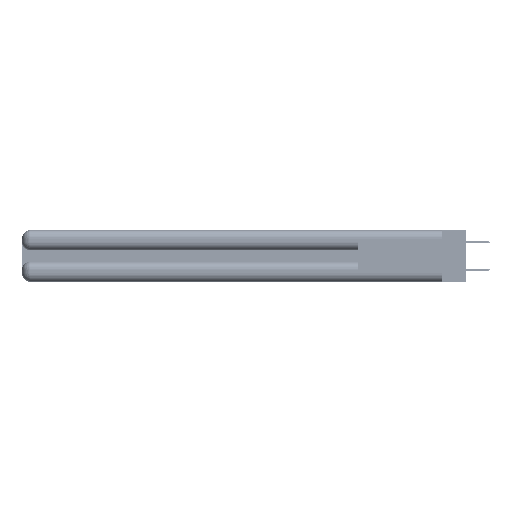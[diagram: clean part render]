
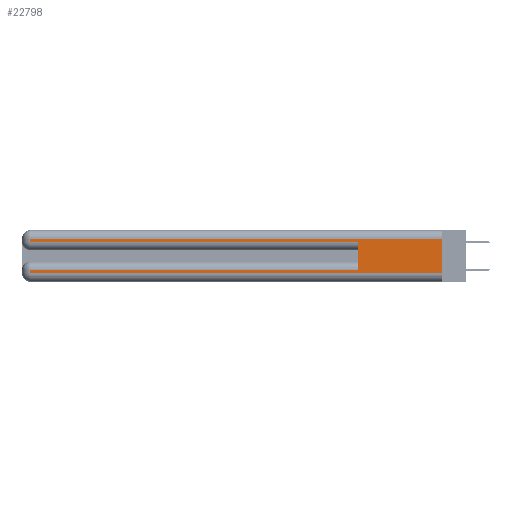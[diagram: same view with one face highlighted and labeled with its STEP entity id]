
A CAD part, left-side view. The second image highlights one B-rep face of the part: STEP entity #22798.
In plain terms, the highlighted planar face has unit normal (-1, 0, 0).
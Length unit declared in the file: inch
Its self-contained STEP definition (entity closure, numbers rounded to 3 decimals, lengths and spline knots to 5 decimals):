
#165 = CARTESIAN_POINT ( 'NONE',  ( 0., 2.94, 0.285 ) ) ;
#1578 = ORIENTED_EDGE ( 'NONE', *, *, #39622, .T. ) ;
#2757 = DIRECTION ( 'NONE',  ( 0., -1., 0. ) ) ;
#2798 = CARTESIAN_POINT ( 'NONE',  ( 0., 0., 0.37 ) ) ;
#3080 = DIRECTION ( 'NONE',  ( 0., 0., -1. ) ) ;
#5945 = ORIENTED_EDGE ( 'NONE', *, *, #26925, .T. ) ;
#6852 = DIRECTION ( 'NONE',  ( 0., 0., -1. ) ) ;
#8112 = ORIENTED_EDGE ( 'NONE', *, *, #46633, .F. ) ;
#8139 = ORIENTED_EDGE ( 'NONE', *, *, #44280, .T. ) ;
#10181 = VERTEX_POINT ( 'NONE', #15805 ) ;
#10468 = DIRECTION ( 'NONE',  ( 1., 0., 0. ) ) ;
#10875 = CARTESIAN_POINT ( 'NONE',  ( 0., 2.94, 0.37 ) ) ;
#11066 = LINE ( 'NONE', #31436, #44846 ) ;
#11734 = LINE ( 'NONE', #26992, #31487 ) ;
#11918 = CARTESIAN_POINT ( 'NONE',  ( 0., 2.94, 0.31 ) ) ;
#14410 = CARTESIAN_POINT ( 'NONE',  ( 0., 0.6, 0.285 ) ) ;
#14662 = VERTEX_POINT ( 'NONE', #48369 ) ;
#14761 = LINE ( 'NONE', #19274, #49781 ) ;
#15805 = CARTESIAN_POINT ( 'NONE',  ( 0., 0.6, 0.085 ) ) ;
#16126 = DIRECTION ( 'NONE',  ( 0., 0., 1. ) ) ;
#17267 = VECTOR ( 'NONE', #28965, 39.37008 ) ;
#17401 = VECTOR ( 'NONE', #46156, 39.37008 ) ;
#19274 = CARTESIAN_POINT ( 'NONE',  ( 0., 2.94, 0.37 ) ) ;
#19809 = VERTEX_POINT ( 'NONE', #11918 ) ;
#20267 = EDGE_CURVE ( 'NONE', #10181, #33226, #32364, .T. ) ;
#21415 = VERTEX_POINT ( 'NONE', #48087 ) ;
#22316 = CARTESIAN_POINT ( 'NONE',  ( 0., 0., 0.06 ) ) ;
#22798 = ADVANCED_FACE ( 'NONE', ( #28886 ), #51208, .F. ) ;
#24554 = ORIENTED_EDGE ( 'NONE', *, *, #32265, .T. ) ;
#25911 = VECTOR ( 'NONE', #47377, 39.37008 ) ;
#26925 = EDGE_CURVE ( 'NONE', #34986, #21415, #50017, .T. ) ;
#26992 = CARTESIAN_POINT ( 'NONE',  ( 0., 0., 0.285 ) ) ;
#28069 = CARTESIAN_POINT ( 'NONE',  ( 0., 0.6, 0.145 ) ) ;
#28886 = FACE_OUTER_BOUND ( 'NONE', #49417, .T. ) ;
#28965 = DIRECTION ( 'NONE',  ( 0., 1., 0. ) ) ;
#30419 = VERTEX_POINT ( 'NONE', #49189 ) ;
#30846 = ORIENTED_EDGE ( 'NONE', *, *, #20267, .F. ) ;
#31436 = CARTESIAN_POINT ( 'NONE',  ( 0., 0., 0.37 ) ) ;
#31487 = VECTOR ( 'NONE', #2757, 39.37008 ) ;
#32265 = EDGE_CURVE ( 'NONE', #42070, #33226, #11734, .T. ) ;
#32364 = LINE ( 'NONE', #28069, #46350 ) ;
#33226 = VERTEX_POINT ( 'NONE', #14410 ) ;
#34199 = LINE ( 'NONE', #10875, #25911 ) ;
#34511 = LINE ( 'NONE', #48033, #17267 ) ;
#34815 = DIRECTION ( 'NONE',  ( 0., -1., 0. ) ) ;
#34986 = VERTEX_POINT ( 'NONE', #44717 ) ;
#35780 = ORIENTED_EDGE ( 'NONE', *, *, #51210, .T. ) ;
#36680 = VECTOR ( 'NONE', #34815, 39.37008 ) ;
#37811 = LINE ( 'NONE', #50227, #17401 ) ;
#38390 = AXIS2_PLACEMENT_3D ( 'NONE', #2798, #10468, #39308 ) ;
#39308 = DIRECTION ( 'NONE',  ( 0., 0., -1. ) ) ;
#39622 = EDGE_CURVE ( 'NONE', #19809, #42070, #14761, .T. ) ;
#42070 = VERTEX_POINT ( 'NONE', #165 ) ;
#42863 = ORIENTED_EDGE ( 'NONE', *, *, #52314, .T. ) ;
#44280 = EDGE_CURVE ( 'NONE', #14662, #34986, #34199, .T. ) ;
#44717 = CARTESIAN_POINT ( 'NONE',  ( 0., 2.94, 0.06 ) ) ;
#44846 = VECTOR ( 'NONE', #6852, 39.37008 ) ;
#46156 = DIRECTION ( 'NONE',  ( 0., 1., 0. ) ) ;
#46350 = VECTOR ( 'NONE', #16126, 39.37008 ) ;
#46633 = EDGE_CURVE ( 'NONE', #30419, #21415, #11066, .T. ) ;
#47377 = DIRECTION ( 'NONE',  ( 0., 0., -1. ) ) ;
#48033 = CARTESIAN_POINT ( 'NONE',  ( 0., 0., 0.31 ) ) ;
#48087 = CARTESIAN_POINT ( 'NONE',  ( 0., 0., 0.06 ) ) ;
#48369 = CARTESIAN_POINT ( 'NONE',  ( 0., 2.94, 0.085 ) ) ;
#49189 = CARTESIAN_POINT ( 'NONE',  ( 0., 0., 0.31 ) ) ;
#49417 = EDGE_LOOP ( 'NONE', ( #8112, #42863, #1578, #24554, #30846, #35780, #8139, #5945 ) ) ;
#49781 = VECTOR ( 'NONE', #3080, 39.37008 ) ;
#50017 = LINE ( 'NONE', #22316, #36680 ) ;
#50227 = CARTESIAN_POINT ( 'NONE',  ( 0., 0., 0.085 ) ) ;
#51208 = PLANE ( 'NONE',  #38390 ) ;
#51210 = EDGE_CURVE ( 'NONE', #10181, #14662, #37811, .T. ) ;
#52314 = EDGE_CURVE ( 'NONE', #30419, #19809, #34511, .T. ) ;
